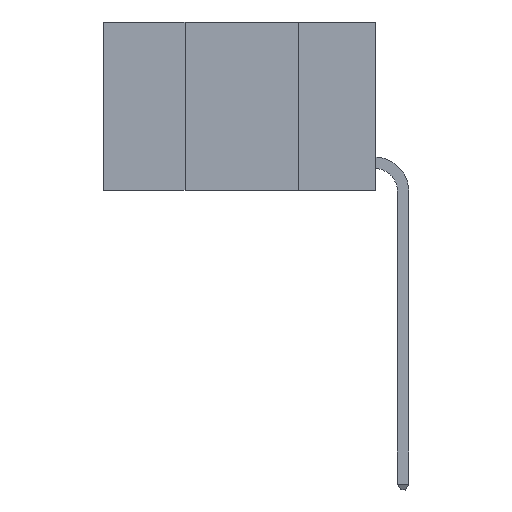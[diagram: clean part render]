
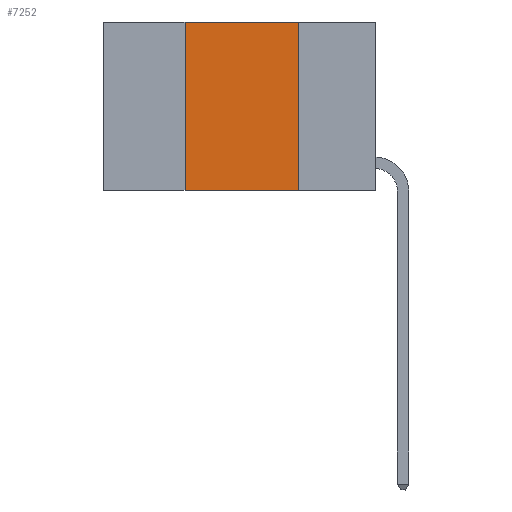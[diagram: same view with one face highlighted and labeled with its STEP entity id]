
A CAD part, left-side view. The second image highlights one B-rep face of the part: STEP entity #7252.
In plain terms, the highlighted planar face has unit normal (-1, 0, 0).
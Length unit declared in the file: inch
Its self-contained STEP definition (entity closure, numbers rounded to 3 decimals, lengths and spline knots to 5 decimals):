
#231 = ORIENTED_EDGE ( 'NONE', *, *, #7858, .F. ) ;
#264 = VECTOR ( 'NONE', #3086, 39.37008 ) ;
#759 = CARTESIAN_POINT ( 'NONE',  ( 0., 0.6, 0. ) ) ;
#1463 = CARTESIAN_POINT ( 'NONE',  ( 0., 0.6, 0. ) ) ;
#1547 = DIRECTION ( 'NONE',  ( 0., 0., -1. ) ) ;
#1771 = DIRECTION ( 'NONE',  ( 0., 0., -1. ) ) ;
#2044 = VECTOR ( 'NONE', #5668, 39.37008 ) ;
#2400 = AXIS2_PLACEMENT_3D ( 'NONE', #759, #6113, #1547 ) ;
#2447 = CARTESIAN_POINT ( 'NONE',  ( 0., 0.17, -0.37 ) ) ;
#2821 = VECTOR ( 'NONE', #1771, 39.37008 ) ;
#3086 = DIRECTION ( 'NONE',  ( 0., -1., 0. ) ) ;
#3208 = VERTEX_POINT ( 'NONE', #2447 ) ;
#3294 = VERTEX_POINT ( 'NONE', #7795 ) ;
#3363 = CARTESIAN_POINT ( 'NONE',  ( 0., 0.42, 0. ) ) ;
#4068 = LINE ( 'NONE', #3363, #2044 ) ;
#4570 = PLANE ( 'NONE',  #2400 ) ;
#4688 = EDGE_CURVE ( 'NONE', #7600, #3294, #4068, .T. ) ;
#5364 = EDGE_CURVE ( 'NONE', #7600, #3208, #6445, .T. ) ;
#5668 = DIRECTION ( 'NONE',  ( 0., 0., 1. ) ) ;
#6113 = DIRECTION ( 'NONE',  ( 1., 0., 0. ) ) ;
#6226 = EDGE_CURVE ( 'NONE', #9682, #3208, #8791, .T. ) ;
#6445 = LINE ( 'NONE', #8337, #264 ) ;
#6502 = LINE ( 'NONE', #1463, #8415 ) ;
#6619 = EDGE_LOOP ( 'NONE', ( #8780, #231, #7912, #8068 ) ) ;
#6800 = DIRECTION ( 'NONE',  ( 0., -1., 0. ) ) ;
#7252 = ADVANCED_FACE ( 'NONE', ( #7852 ), #4570, .F. ) ;
#7600 = VERTEX_POINT ( 'NONE', #9351 ) ;
#7795 = CARTESIAN_POINT ( 'NONE',  ( 0., 0.42, 0. ) ) ;
#7852 = FACE_OUTER_BOUND ( 'NONE', #6619, .T. ) ;
#7858 = EDGE_CURVE ( 'NONE', #3294, #9682, #6502, .T. ) ;
#7912 = ORIENTED_EDGE ( 'NONE', *, *, #4688, .F. ) ;
#8068 = ORIENTED_EDGE ( 'NONE', *, *, #5364, .T. ) ;
#8148 = CARTESIAN_POINT ( 'NONE',  ( 0., 0.17, 0. ) ) ;
#8337 = CARTESIAN_POINT ( 'NONE',  ( 0., 0.6, -0.37 ) ) ;
#8415 = VECTOR ( 'NONE', #6800, 39.37008 ) ;
#8780 = ORIENTED_EDGE ( 'NONE', *, *, #6226, .F. ) ;
#8791 = LINE ( 'NONE', #9204, #2821 ) ;
#9204 = CARTESIAN_POINT ( 'NONE',  ( 0., 0.17, 0. ) ) ;
#9351 = CARTESIAN_POINT ( 'NONE',  ( 0., 0.42, -0.37 ) ) ;
#9682 = VERTEX_POINT ( 'NONE', #8148 ) ;
